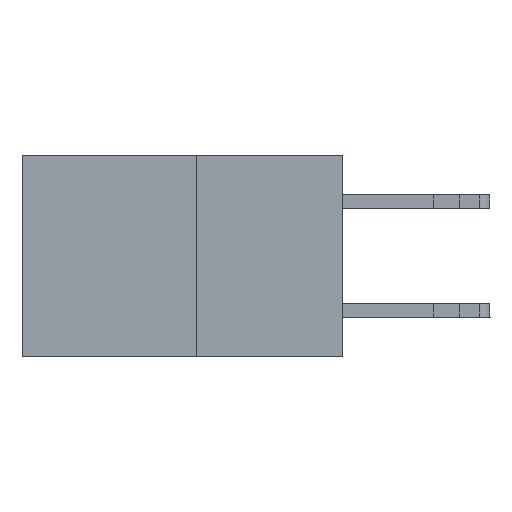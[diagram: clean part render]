
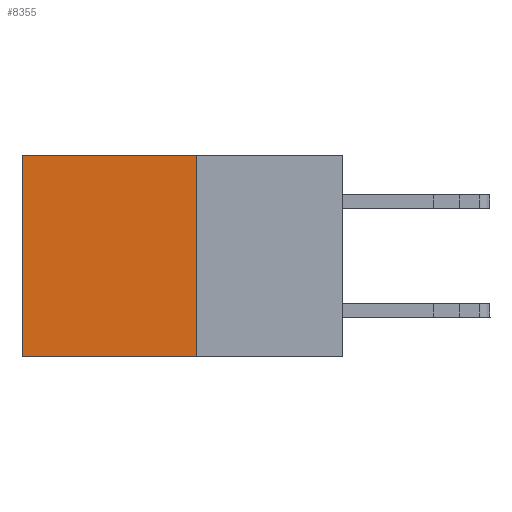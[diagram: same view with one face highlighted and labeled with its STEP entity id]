
A CAD part, left-side view. The second image highlights one B-rep face of the part: STEP entity #8355.
In plain terms, the highlighted planar face has unit normal (-1, 0, 0).
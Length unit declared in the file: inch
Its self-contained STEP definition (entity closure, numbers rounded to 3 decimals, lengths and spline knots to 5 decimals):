
#372 = VECTOR ( 'NONE', #13545, 39.37008 ) ;
#2371 = ORIENTED_EDGE ( 'NONE', *, *, #16360, .T. ) ;
#2947 = EDGE_CURVE ( 'NONE', #6406, #12945, #3147, .T. ) ;
#3147 = LINE ( 'NONE', #25449, #21840 ) ;
#3596 = LINE ( 'NONE', #14925, #15355 ) ;
#3680 = ORIENTED_EDGE ( 'NONE', *, *, #2947, .F. ) ;
#4088 = VECTOR ( 'NONE', #5622, 39.37008 ) ;
#4532 = DIRECTION ( 'NONE',  ( 1., 0., 0. ) ) ;
#4560 = ORIENTED_EDGE ( 'NONE', *, *, #6583, .F. ) ;
#5622 = DIRECTION ( 'NONE',  ( 0., 1., 0. ) ) ;
#6406 = VERTEX_POINT ( 'NONE', #18030 ) ;
#6583 = EDGE_CURVE ( 'NONE', #12945, #27797, #25155, .T. ) ;
#8355 = ADVANCED_FACE ( 'NONE', ( #19835 ), #9067, .F. ) ;
#8703 = VERTEX_POINT ( 'NONE', #10499 ) ;
#9067 = PLANE ( 'NONE',  #22150 ) ;
#10499 = CARTESIAN_POINT ( 'NONE',  ( 0.277, 0.59, 0. ) ) ;
#12945 = VERTEX_POINT ( 'NONE', #19770 ) ;
#13207 = ORIENTED_EDGE ( 'NONE', *, *, #24770, .T. ) ;
#13545 = DIRECTION ( 'NONE',  ( 0., 1., 0. ) ) ;
#13745 = CARTESIAN_POINT ( 'NONE',  ( 0.277, 0.27, -0.37 ) ) ;
#14925 = CARTESIAN_POINT ( 'NONE',  ( 0.277, 0.59, -0.37 ) ) ;
#15355 = VECTOR ( 'NONE', #17285, 39.37008 ) ;
#16233 = CARTESIAN_POINT ( 'NONE',  ( 0.277, 0.27, -0.37 ) ) ;
#16360 = EDGE_CURVE ( 'NONE', #6406, #8703, #23448, .T. ) ;
#17285 = DIRECTION ( 'NONE',  ( 0., 0., -1. ) ) ;
#18030 = CARTESIAN_POINT ( 'NONE',  ( 0.277, 0.27, 0. ) ) ;
#19770 = CARTESIAN_POINT ( 'NONE',  ( 0.277, 0.27, -0.37 ) ) ;
#19835 = FACE_OUTER_BOUND ( 'NONE', #28406, .T. ) ;
#20902 = DIRECTION ( 'NONE',  ( 0., 0., -1. ) ) ;
#21840 = VECTOR ( 'NONE', #24075, 39.37008 ) ;
#21973 = CARTESIAN_POINT ( 'NONE',  ( 0.277, 0.27, 0. ) ) ;
#22150 = AXIS2_PLACEMENT_3D ( 'NONE', #16233, #4532, #20902 ) ;
#23448 = LINE ( 'NONE', #21973, #4088 ) ;
#24075 = DIRECTION ( 'NONE',  ( 0., 0., -1. ) ) ;
#24770 = EDGE_CURVE ( 'NONE', #8703, #27797, #3596, .T. ) ;
#25155 = LINE ( 'NONE', #13745, #372 ) ;
#25449 = CARTESIAN_POINT ( 'NONE',  ( 0.277, 0.27, -0.37 ) ) ;
#27797 = VERTEX_POINT ( 'NONE', #29272 ) ;
#28406 = EDGE_LOOP ( 'NONE', ( #13207, #4560, #3680, #2371 ) ) ;
#29272 = CARTESIAN_POINT ( 'NONE',  ( 0.277, 0.59, -0.37 ) ) ;
